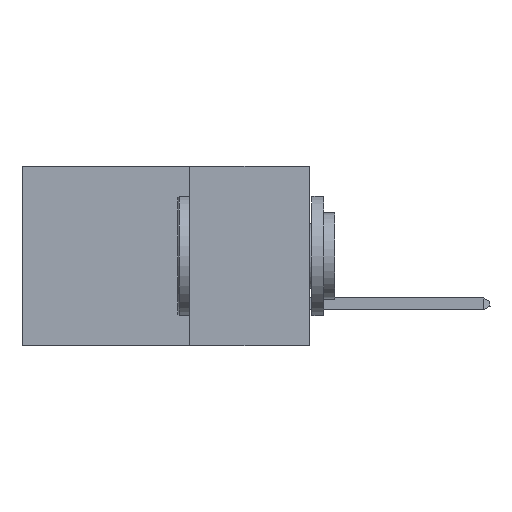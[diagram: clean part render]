
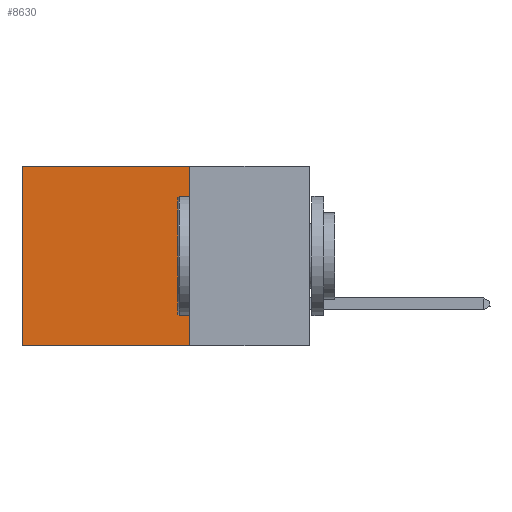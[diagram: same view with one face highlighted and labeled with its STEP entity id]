
A CAD part, left-side view. The second image highlights one B-rep face of the part: STEP entity #8630.
In plain terms, the highlighted planar face has unit normal (-1, 0, 0).
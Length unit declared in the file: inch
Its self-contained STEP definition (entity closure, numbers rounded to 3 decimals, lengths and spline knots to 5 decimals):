
#44 = AXIS2_PLACEMENT_3D ( 'NONE', #16801, #5306, #6816 ) ;
#635 = LINE ( 'NONE', #18034, #17809 ) ;
#1280 = DIRECTION ( 'NONE',  ( 0., 1., 0. ) ) ;
#1855 = FACE_OUTER_BOUND ( 'NONE', #6922, .T. ) ;
#2080 = DIRECTION ( 'NONE',  ( 0., 0., -1. ) ) ;
#2287 = CARTESIAN_POINT ( 'NONE',  ( 0.2875, 0.25, 0. ) ) ;
#2366 = VERTEX_POINT ( 'NONE', #21173 ) ;
#2393 = VECTOR ( 'NONE', #11581, 39.37008 ) ;
#5306 = DIRECTION ( 'NONE',  ( 1., 0., 0. ) ) ;
#6242 = VERTEX_POINT ( 'NONE', #10461 ) ;
#6816 = DIRECTION ( 'NONE',  ( 0., 0., -1. ) ) ;
#6922 = EDGE_LOOP ( 'NONE', ( #10790, #16845, #7852, #16799 ) ) ;
#7748 = CARTESIAN_POINT ( 'NONE',  ( 0.2875, 0.6, 0. ) ) ;
#7852 = ORIENTED_EDGE ( 'NONE', *, *, #20284, .F. ) ;
#8630 = ADVANCED_FACE ( 'NONE', ( #1855 ), #11900, .F. ) ;
#8657 = CARTESIAN_POINT ( 'NONE',  ( 0.2875, 0.25, -0.375 ) ) ;
#10066 = VERTEX_POINT ( 'NONE', #7748 ) ;
#10461 = CARTESIAN_POINT ( 'NONE',  ( 0.2875, 0.6, -0.375 ) ) ;
#10607 = DIRECTION ( 'NONE',  ( 0., 1., 0. ) ) ;
#10790 = ORIENTED_EDGE ( 'NONE', *, *, #14930, .T. ) ;
#11581 = DIRECTION ( 'NONE',  ( 0., 0., -1. ) ) ;
#11750 = LINE ( 'NONE', #8657, #13336 ) ;
#11900 = PLANE ( 'NONE',  #44 ) ;
#11967 = VECTOR ( 'NONE', #10607, 39.37008 ) ;
#13336 = VECTOR ( 'NONE', #2080, 39.37008 ) ;
#14354 = LINE ( 'NONE', #16348, #2393 ) ;
#14662 = VERTEX_POINT ( 'NONE', #2287 ) ;
#14930 = EDGE_CURVE ( 'NONE', #10066, #6242, #14354, .T. ) ;
#16348 = CARTESIAN_POINT ( 'NONE',  ( 0.2875, 0.6, -0.375 ) ) ;
#16799 = ORIENTED_EDGE ( 'NONE', *, *, #21284, .T. ) ;
#16801 = CARTESIAN_POINT ( 'NONE',  ( 0.2875, 0.25, -0.375 ) ) ;
#16845 = ORIENTED_EDGE ( 'NONE', *, *, #19943, .F. ) ;
#17809 = VECTOR ( 'NONE', #1280, 39.37008 ) ;
#18034 = CARTESIAN_POINT ( 'NONE',  ( 0.2875, 0.25, -0.375 ) ) ;
#19567 = LINE ( 'NONE', #20781, #11967 ) ;
#19943 = EDGE_CURVE ( 'NONE', #2366, #6242, #635, .T. ) ;
#20284 = EDGE_CURVE ( 'NONE', #14662, #2366, #11750, .T. ) ;
#20781 = CARTESIAN_POINT ( 'NONE',  ( 0.2875, 0.25, 0. ) ) ;
#21173 = CARTESIAN_POINT ( 'NONE',  ( 0.2875, 0.25, -0.375 ) ) ;
#21284 = EDGE_CURVE ( 'NONE', #14662, #10066, #19567, .T. ) ;
